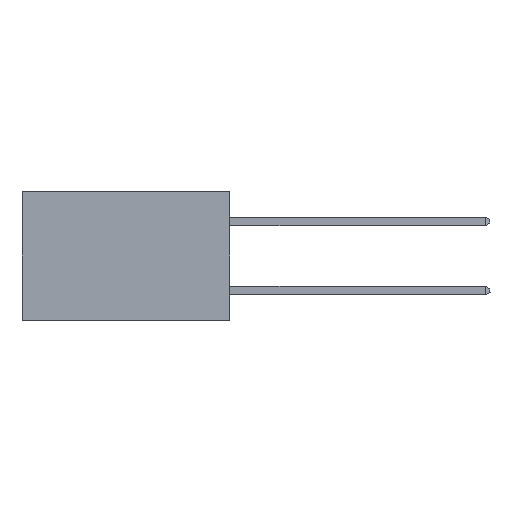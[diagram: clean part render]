
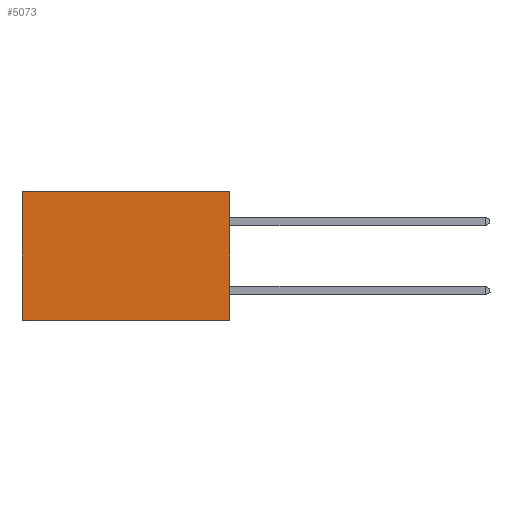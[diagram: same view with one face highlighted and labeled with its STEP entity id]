
A CAD part, left-side view. The second image highlights one B-rep face of the part: STEP entity #5073.
In plain terms, the highlighted planar face has unit normal (-1, 0, 0).
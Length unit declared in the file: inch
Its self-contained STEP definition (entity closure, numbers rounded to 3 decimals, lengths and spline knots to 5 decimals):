
#720 = VECTOR ( 'NONE', #3684, 39.37008 ) ;
#783 = DIRECTION ( 'NONE',  ( 0., 1., 0. ) ) ;
#1337 = EDGE_CURVE ( 'NONE', #4653, #4031, #5266, .T. ) ;
#1449 = CARTESIAN_POINT ( 'NONE',  ( 0.298, 0., -0.37 ) ) ;
#1699 = EDGE_CURVE ( 'NONE', #4653, #9207, #1865, .T. ) ;
#1865 = LINE ( 'NONE', #3520, #720 ) ;
#2058 = CARTESIAN_POINT ( 'NONE',  ( 0.298, 0.6, 0. ) ) ;
#2180 = EDGE_CURVE ( 'NONE', #9207, #3243, #6652, .T. ) ;
#2338 = ORIENTED_EDGE ( 'NONE', *, *, #2180, .T. ) ;
#2661 = ORIENTED_EDGE ( 'NONE', *, *, #6791, .F. ) ;
#3046 = CARTESIAN_POINT ( 'NONE',  ( 0.298, 0., 0. ) ) ;
#3192 = VECTOR ( 'NONE', #6663, 39.37008 ) ;
#3243 = VERTEX_POINT ( 'NONE', #9434 ) ;
#3262 = VECTOR ( 'NONE', #783, 39.37008 ) ;
#3334 = VECTOR ( 'NONE', #3447, 39.37008 ) ;
#3447 = DIRECTION ( 'NONE',  ( 0., 0., -1. ) ) ;
#3510 = FACE_OUTER_BOUND ( 'NONE', #6755, .T. ) ;
#3520 = CARTESIAN_POINT ( 'NONE',  ( 0.298, 0., 0. ) ) ;
#3684 = DIRECTION ( 'NONE',  ( 0., 1., 0. ) ) ;
#3810 = DIRECTION ( 'NONE',  ( 1., 0., 0. ) ) ;
#4031 = VERTEX_POINT ( 'NONE', #6442 ) ;
#4653 = VERTEX_POINT ( 'NONE', #9219 ) ;
#5073 = ADVANCED_FACE ( 'NONE', ( #3510 ), #5259, .F. ) ;
#5259 = PLANE ( 'NONE',  #6261 ) ;
#5266 = LINE ( 'NONE', #5844, #3192 ) ;
#5844 = CARTESIAN_POINT ( 'NONE',  ( 0.298, 0., 0. ) ) ;
#6261 = AXIS2_PLACEMENT_3D ( 'NONE', #3046, #3810, #8170 ) ;
#6289 = ORIENTED_EDGE ( 'NONE', *, *, #1337, .F. ) ;
#6442 = CARTESIAN_POINT ( 'NONE',  ( 0.298, 0., -0.37 ) ) ;
#6533 = ORIENTED_EDGE ( 'NONE', *, *, #1699, .T. ) ;
#6652 = LINE ( 'NONE', #2058, #3334 ) ;
#6663 = DIRECTION ( 'NONE',  ( 0., 0., -1. ) ) ;
#6755 = EDGE_LOOP ( 'NONE', ( #2338, #2661, #6289, #6533 ) ) ;
#6791 = EDGE_CURVE ( 'NONE', #4031, #3243, #7852, .T. ) ;
#7852 = LINE ( 'NONE', #1449, #3262 ) ;
#8081 = CARTESIAN_POINT ( 'NONE',  ( 0.298, 0.6, 0. ) ) ;
#8170 = DIRECTION ( 'NONE',  ( 0., 0., -1. ) ) ;
#9207 = VERTEX_POINT ( 'NONE', #8081 ) ;
#9219 = CARTESIAN_POINT ( 'NONE',  ( 0.298, 0., 0. ) ) ;
#9434 = CARTESIAN_POINT ( 'NONE',  ( 0.298, 0.6, -0.37 ) ) ;
